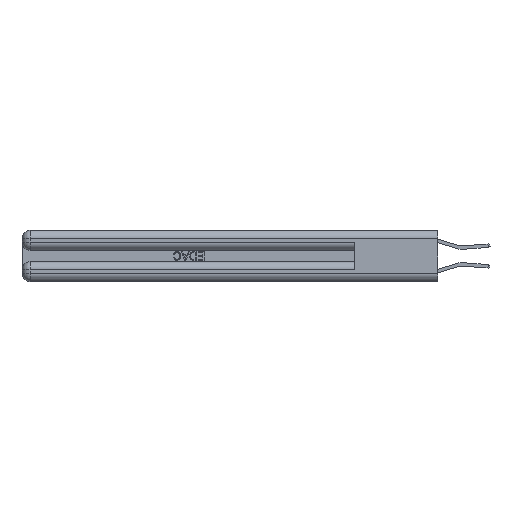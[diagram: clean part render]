
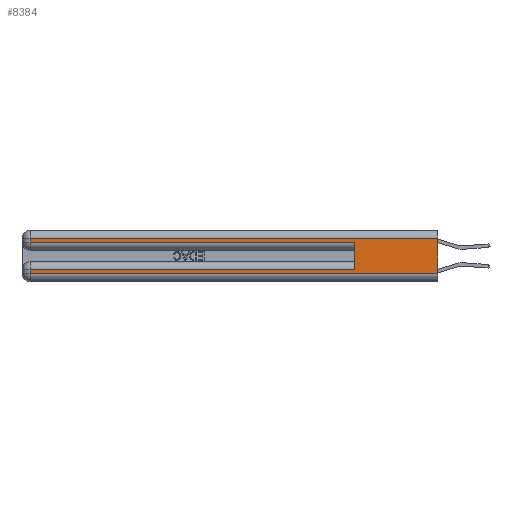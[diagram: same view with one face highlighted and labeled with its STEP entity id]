
A CAD part, left-side view. The second image highlights one B-rep face of the part: STEP entity #8384.
In plain terms, the highlighted planar face has unit normal (-1, 0, 0).
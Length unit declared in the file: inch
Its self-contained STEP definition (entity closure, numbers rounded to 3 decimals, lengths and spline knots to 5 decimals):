
#63 = LINE ( 'NONE', #25839, #1918 ) ;
#263 = LINE ( 'NONE', #9862, #13091 ) ;
#282 = LINE ( 'NONE', #19304, #19948 ) ;
#895 = CARTESIAN_POINT ( 'NONE',  ( 0., 2.94, 0.06 ) ) ;
#1117 = LINE ( 'NONE', #3962, #10533 ) ;
#1918 = VECTOR ( 'NONE', #28365, 39.37008 ) ;
#3648 = DIRECTION ( 'NONE',  ( 0., 0., -1. ) ) ;
#3754 = CARTESIAN_POINT ( 'NONE',  ( 0., 0., 0.37 ) ) ;
#3962 = CARTESIAN_POINT ( 'NONE',  ( 0., 2.94, 0.37 ) ) ;
#4419 = ORIENTED_EDGE ( 'NONE', *, *, #23156, .T. ) ;
#5450 = CARTESIAN_POINT ( 'NONE',  ( 0., 0., 0.37 ) ) ;
#5528 = EDGE_CURVE ( 'NONE', #22453, #11012, #282, .T. ) ;
#6192 = VECTOR ( 'NONE', #10782, 39.37008 ) ;
#6261 = ORIENTED_EDGE ( 'NONE', *, *, #30245, .F. ) ;
#6371 = AXIS2_PLACEMENT_3D ( 'NONE', #3754, #25431, #6716 ) ;
#6716 = DIRECTION ( 'NONE',  ( 0., 0., -1. ) ) ;
#7079 = CARTESIAN_POINT ( 'NONE',  ( 0., 2.94, 0.085 ) ) ;
#7494 = DIRECTION ( 'NONE',  ( 0., 1., 0. ) ) ;
#7933 = VECTOR ( 'NONE', #27486, 39.37008 ) ;
#8254 = LINE ( 'NONE', #17867, #6192 ) ;
#8384 = ADVANCED_FACE ( 'NONE', ( #12700 ), #22285, .F. ) ;
#9623 = VECTOR ( 'NONE', #11920, 39.37008 ) ;
#9862 = CARTESIAN_POINT ( 'NONE',  ( 0., 0., 0.085 ) ) ;
#10106 = ORIENTED_EDGE ( 'NONE', *, *, #23344, .T. ) ;
#10533 = VECTOR ( 'NONE', #3648, 39.37008 ) ;
#10782 = DIRECTION ( 'NONE',  ( 0., 0., 1. ) ) ;
#11012 = VERTEX_POINT ( 'NONE', #22623 ) ;
#11226 = ORIENTED_EDGE ( 'NONE', *, *, #25894, .T. ) ;
#11663 = LINE ( 'NONE', #26262, #16933 ) ;
#11920 = DIRECTION ( 'NONE',  ( 0., 0., -1. ) ) ;
#11921 = VERTEX_POINT ( 'NONE', #20036 ) ;
#12470 = ORIENTED_EDGE ( 'NONE', *, *, #5528, .T. ) ;
#12700 = FACE_OUTER_BOUND ( 'NONE', #14914, .T. ) ;
#13091 = VECTOR ( 'NONE', #7494, 39.37008 ) ;
#14198 = VERTEX_POINT ( 'NONE', #21340 ) ;
#14370 = VERTEX_POINT ( 'NONE', #895 ) ;
#14726 = CARTESIAN_POINT ( 'NONE',  ( 0., 2.94, 0.31 ) ) ;
#14914 = EDGE_LOOP ( 'NONE', ( #21765, #28658, #12470, #10106, #6261, #11226, #30231, #4419 ) ) ;
#14951 = VERTEX_POINT ( 'NONE', #7079 ) ;
#15277 = CARTESIAN_POINT ( 'NONE',  ( 0., 0., 0.06 ) ) ;
#16933 = VECTOR ( 'NONE', #28485, 39.37008 ) ;
#17586 = CARTESIAN_POINT ( 'NONE',  ( 0., 0., 0.285 ) ) ;
#17867 = CARTESIAN_POINT ( 'NONE',  ( 0., 0.6, 0.145 ) ) ;
#19304 = CARTESIAN_POINT ( 'NONE',  ( 0., 2.94, 0.37 ) ) ;
#19948 = VECTOR ( 'NONE', #24330, 39.37008 ) ;
#20036 = CARTESIAN_POINT ( 'NONE',  ( 0., 0.6, 0.085 ) ) ;
#21340 = CARTESIAN_POINT ( 'NONE',  ( 0., 0.6, 0.285 ) ) ;
#21703 = VERTEX_POINT ( 'NONE', #27825 ) ;
#21765 = ORIENTED_EDGE ( 'NONE', *, *, #27252, .F. ) ;
#22285 = PLANE ( 'NONE',  #6371 ) ;
#22287 = LINE ( 'NONE', #17586, #7933 ) ;
#22453 = VERTEX_POINT ( 'NONE', #14726 ) ;
#22623 = CARTESIAN_POINT ( 'NONE',  ( 0., 2.94, 0.285 ) ) ;
#22799 = EDGE_CURVE ( 'NONE', #21703, #22453, #63, .T. ) ;
#23156 = EDGE_CURVE ( 'NONE', #14370, #28403, #11663, .T. ) ;
#23344 = EDGE_CURVE ( 'NONE', #11012, #14198, #22287, .T. ) ;
#24330 = DIRECTION ( 'NONE',  ( 0., 0., -1. ) ) ;
#24723 = EDGE_CURVE ( 'NONE', #14951, #14370, #1117, .T. ) ;
#25431 = DIRECTION ( 'NONE',  ( 1., 0., 0. ) ) ;
#25839 = CARTESIAN_POINT ( 'NONE',  ( 0., 0., 0.31 ) ) ;
#25894 = EDGE_CURVE ( 'NONE', #11921, #14951, #263, .T. ) ;
#26262 = CARTESIAN_POINT ( 'NONE',  ( 0., 0., 0.06 ) ) ;
#26822 = LINE ( 'NONE', #5450, #9623 ) ;
#27252 = EDGE_CURVE ( 'NONE', #21703, #28403, #26822, .T. ) ;
#27486 = DIRECTION ( 'NONE',  ( 0., -1., 0. ) ) ;
#27825 = CARTESIAN_POINT ( 'NONE',  ( 0., 0., 0.31 ) ) ;
#28365 = DIRECTION ( 'NONE',  ( 0., 1., 0. ) ) ;
#28403 = VERTEX_POINT ( 'NONE', #15277 ) ;
#28485 = DIRECTION ( 'NONE',  ( 0., -1., 0. ) ) ;
#28658 = ORIENTED_EDGE ( 'NONE', *, *, #22799, .T. ) ;
#30231 = ORIENTED_EDGE ( 'NONE', *, *, #24723, .T. ) ;
#30245 = EDGE_CURVE ( 'NONE', #11921, #14198, #8254, .T. ) ;
